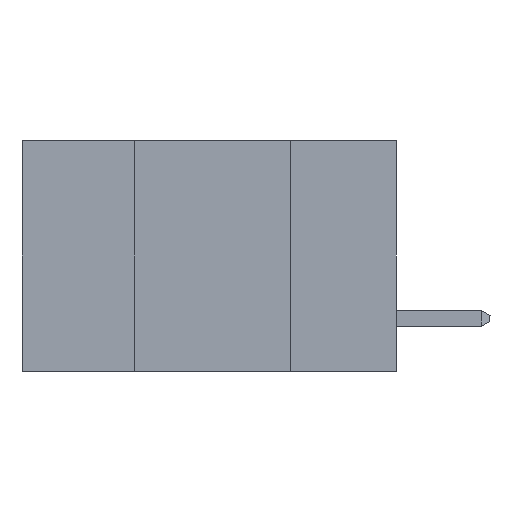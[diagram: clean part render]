
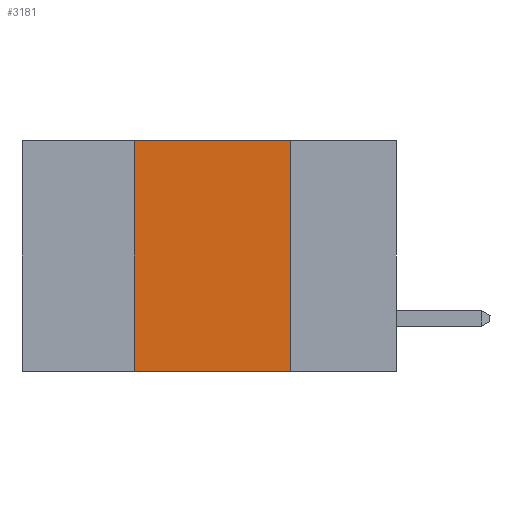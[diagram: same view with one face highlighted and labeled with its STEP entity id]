
A CAD part, left-side view. The second image highlights one B-rep face of the part: STEP entity #3181.
In plain terms, the highlighted planar face has unit normal (-1, 0, 0).
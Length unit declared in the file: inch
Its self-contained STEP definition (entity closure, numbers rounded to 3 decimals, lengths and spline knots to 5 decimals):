
#88 = ORIENTED_EDGE ( 'NONE', *, *, #7449, .F. ) ;
#290 = ORIENTED_EDGE ( 'NONE', *, *, #6799, .F. ) ;
#423 = ORIENTED_EDGE ( 'NONE', *, *, #6124, .T. ) ;
#490 = DIRECTION ( 'NONE',  ( 0., -1., 0. ) ) ;
#2201 = VECTOR ( 'NONE', #13007, 39.37008 ) ;
#2692 = LINE ( 'NONE', #6864, #7845 ) ;
#2823 = DIRECTION ( 'NONE',  ( 1., 0., 0. ) ) ;
#2857 = VECTOR ( 'NONE', #6850, 39.37008 ) ;
#3181 = ADVANCED_FACE ( 'NONE', ( #4120 ), #12657, .F. ) ;
#3312 = AXIS2_PLACEMENT_3D ( 'NONE', #4978, #2823, #9874 ) ;
#4098 = VERTEX_POINT ( 'NONE', #9350 ) ;
#4120 = FACE_OUTER_BOUND ( 'NONE', #7297, .T. ) ;
#4188 = DIRECTION ( 'NONE',  ( 0., -1., 0. ) ) ;
#4222 = VECTOR ( 'NONE', #4188, 39.37008 ) ;
#4725 = VERTEX_POINT ( 'NONE', #9785 ) ;
#4978 = CARTESIAN_POINT ( 'NONE',  ( 0., 0.6, 0. ) ) ;
#5364 = CARTESIAN_POINT ( 'NONE',  ( 0., 0.42, -0.37 ) ) ;
#5527 = VERTEX_POINT ( 'NONE', #11045 ) ;
#5840 = CARTESIAN_POINT ( 'NONE',  ( 0., 0.17, -0.37 ) ) ;
#6124 = EDGE_CURVE ( 'NONE', #5527, #11290, #10029, .T. ) ;
#6799 = EDGE_CURVE ( 'NONE', #5527, #4098, #10259, .T. ) ;
#6850 = DIRECTION ( 'NONE',  ( 0., 0., -1. ) ) ;
#6864 = CARTESIAN_POINT ( 'NONE',  ( 0., 0.6, 0. ) ) ;
#7297 = EDGE_LOOP ( 'NONE', ( #8806, #88, #290, #423 ) ) ;
#7449 = EDGE_CURVE ( 'NONE', #4098, #4725, #2692, .T. ) ;
#7845 = VECTOR ( 'NONE', #490, 39.37008 ) ;
#8074 = EDGE_CURVE ( 'NONE', #4725, #11290, #8266, .T. ) ;
#8266 = LINE ( 'NONE', #5840, #2857 ) ;
#8806 = ORIENTED_EDGE ( 'NONE', *, *, #8074, .F. ) ;
#9350 = CARTESIAN_POINT ( 'NONE',  ( 0., 0.42, 0. ) ) ;
#9785 = CARTESIAN_POINT ( 'NONE',  ( 0., 0.17, 0. ) ) ;
#9874 = DIRECTION ( 'NONE',  ( 0., 0., -1. ) ) ;
#10029 = LINE ( 'NONE', #10985, #4222 ) ;
#10259 = LINE ( 'NONE', #5364, #2201 ) ;
#10985 = CARTESIAN_POINT ( 'NONE',  ( 0., 0.6, -0.37 ) ) ;
#11045 = CARTESIAN_POINT ( 'NONE',  ( 0., 0.42, -0.37 ) ) ;
#11290 = VERTEX_POINT ( 'NONE', #11521 ) ;
#11521 = CARTESIAN_POINT ( 'NONE',  ( 0., 0.17, -0.37 ) ) ;
#12657 = PLANE ( 'NONE',  #3312 ) ;
#13007 = DIRECTION ( 'NONE',  ( 0., 0., 1. ) ) ;
